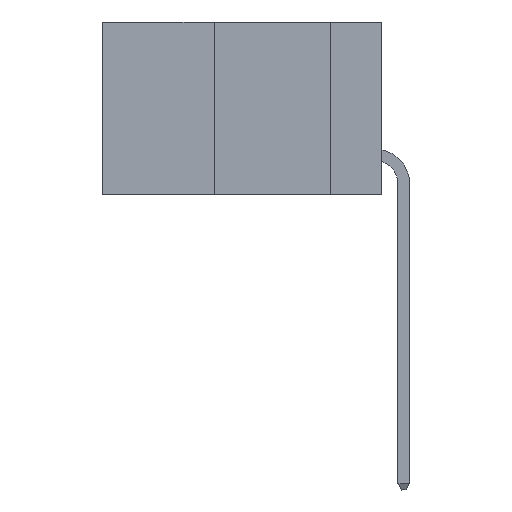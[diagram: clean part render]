
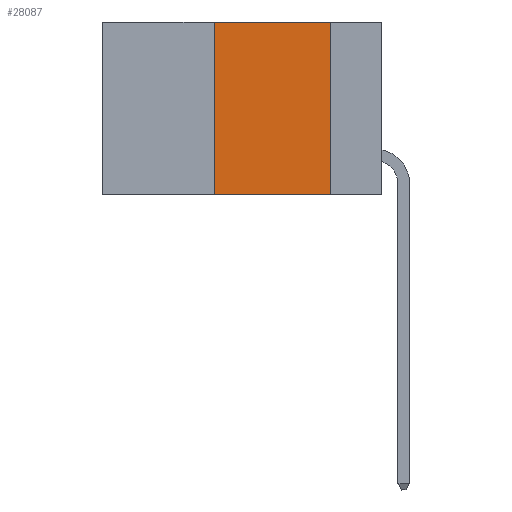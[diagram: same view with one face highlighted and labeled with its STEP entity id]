
A CAD part, left-side view. The second image highlights one B-rep face of the part: STEP entity #28087.
In plain terms, the highlighted planar face has unit normal (-1, 0, 0).
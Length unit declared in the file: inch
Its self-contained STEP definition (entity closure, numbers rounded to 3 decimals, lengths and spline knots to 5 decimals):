
#320 = VERTEX_POINT ( 'NONE', #9743 ) ;
#1239 = DIRECTION ( 'NONE',  ( 0., 0., -1. ) ) ;
#1440 = FACE_OUTER_BOUND ( 'NONE', #11086, .T. ) ;
#2089 = ORIENTED_EDGE ( 'NONE', *, *, #30532, .T. ) ;
#2404 = CARTESIAN_POINT ( 'NONE',  ( 0., 0.36, -0.37 ) ) ;
#4331 = EDGE_CURVE ( 'NONE', #4720, #320, #5184, .T. ) ;
#4720 = VERTEX_POINT ( 'NONE', #30597 ) ;
#5184 = LINE ( 'NONE', #35505, #10340 ) ;
#5500 = EDGE_CURVE ( 'NONE', #20315, #40650, #27942, .T. ) ;
#8812 = CARTESIAN_POINT ( 'NONE',  ( 0., 0.36, 0. ) ) ;
#9072 = CARTESIAN_POINT ( 'NONE',  ( 0., 0.6, 0. ) ) ;
#9743 = CARTESIAN_POINT ( 'NONE',  ( 0., 0.11, -0.37 ) ) ;
#10340 = VECTOR ( 'NONE', #31229, 39.37008 ) ;
#11086 = EDGE_LOOP ( 'NONE', ( #26188, #31780, #42921, #2089 ) ) ;
#11229 = CARTESIAN_POINT ( 'NONE',  ( 0., 0.36, 0. ) ) ;
#11989 = EDGE_CURVE ( 'NONE', #40650, #4720, #20234, .T. ) ;
#12272 = DIRECTION ( 'NONE',  ( 1., 0., 0. ) ) ;
#18130 = DIRECTION ( 'NONE',  ( 0., -1., 0. ) ) ;
#20234 = LINE ( 'NONE', #43416, #45842 ) ;
#20315 = VERTEX_POINT ( 'NONE', #2404 ) ;
#21689 = CARTESIAN_POINT ( 'NONE',  ( 0., 0.6, -0.37 ) ) ;
#23133 = PLANE ( 'NONE',  #43401 ) ;
#26188 = ORIENTED_EDGE ( 'NONE', *, *, #4331, .F. ) ;
#27942 = LINE ( 'NONE', #8812, #32496 ) ;
#28087 = ADVANCED_FACE ( 'NONE', ( #1440 ), #23133, .F. ) ;
#30532 = EDGE_CURVE ( 'NONE', #20315, #320, #33776, .T. ) ;
#30597 = CARTESIAN_POINT ( 'NONE',  ( 0., 0.11, 0. ) ) ;
#31229 = DIRECTION ( 'NONE',  ( 0., 0., -1. ) ) ;
#31780 = ORIENTED_EDGE ( 'NONE', *, *, #11989, .F. ) ;
#32496 = VECTOR ( 'NONE', #34340, 39.37008 ) ;
#33776 = LINE ( 'NONE', #21689, #38339 ) ;
#34340 = DIRECTION ( 'NONE',  ( 0., 0., 1. ) ) ;
#35505 = CARTESIAN_POINT ( 'NONE',  ( 0., 0.11, 0. ) ) ;
#36944 = DIRECTION ( 'NONE',  ( 0., -1., 0. ) ) ;
#38339 = VECTOR ( 'NONE', #36944, 39.37008 ) ;
#40650 = VERTEX_POINT ( 'NONE', #11229 ) ;
#42921 = ORIENTED_EDGE ( 'NONE', *, *, #5500, .F. ) ;
#43401 = AXIS2_PLACEMENT_3D ( 'NONE', #9072, #12272, #1239 ) ;
#43416 = CARTESIAN_POINT ( 'NONE',  ( 0., 0.6, 0. ) ) ;
#45842 = VECTOR ( 'NONE', #18130, 39.37008 ) ;
